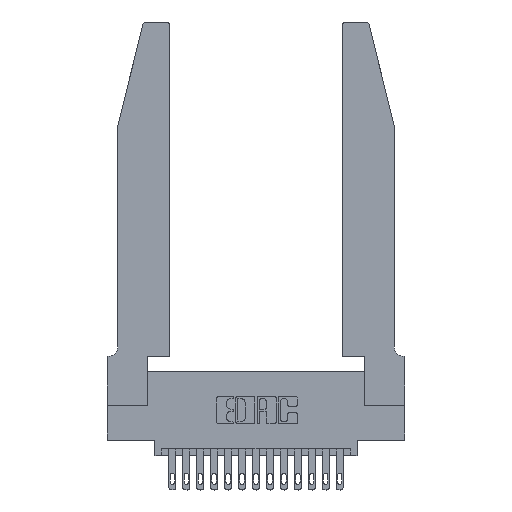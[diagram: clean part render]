
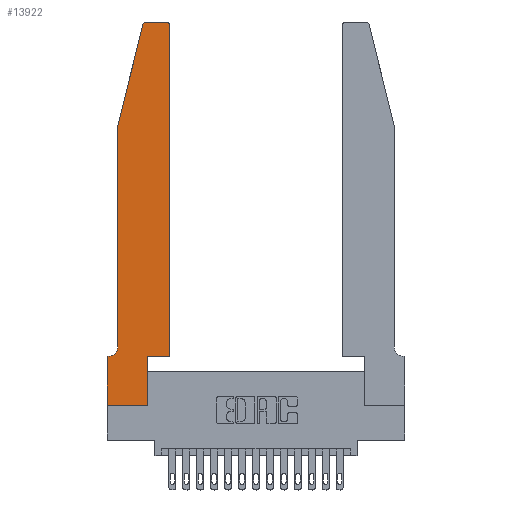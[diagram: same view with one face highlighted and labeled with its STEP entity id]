
A CAD part, top view. The second image highlights one B-rep face of the part: STEP entity #13922.
In plain terms, the highlighted planar face has unit normal (0, 0, 1).
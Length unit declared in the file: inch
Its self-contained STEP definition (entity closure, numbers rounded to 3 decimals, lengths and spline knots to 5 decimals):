
#42 = CARTESIAN_POINT ( 'NONE',  ( 0.25487, 2.72718, 0.37 ) ) ;
#198 = EDGE_LOOP ( 'NONE', ( #1298, #3548, #8835, #11519, #1738, #9997, #5464, #5388, #15684, #5136, #5292, #12281 ) ) ;
#418 = CARTESIAN_POINT ( 'NONE',  ( 0.0755, 2., 0.37 ) ) ;
#589 = VECTOR ( 'NONE', #10722, 39.37008 ) ;
#644 = VERTEX_POINT ( 'NONE', #4199 ) ;
#688 = VERTEX_POINT ( 'NONE', #10249 ) ;
#1087 = DIRECTION ( 'NONE',  ( 0., -1., 0. ) ) ;
#1140 = CARTESIAN_POINT ( 'NONE',  ( 0.4505, 0.35, 0.37 ) ) ;
#1259 = LINE ( 'NONE', #418, #589 ) ;
#1298 = ORIENTED_EDGE ( 'NONE', *, *, #5719, .T. ) ;
#1547 = AXIS2_PLACEMENT_3D ( 'NONE', #6113, #16188, #14755 ) ;
#1638 = LINE ( 'NONE', #12558, #17407 ) ;
#1664 = VECTOR ( 'NONE', #8666, 39.37008 ) ;
#1738 = ORIENTED_EDGE ( 'NONE', *, *, #2951, .T. ) ;
#1989 = CARTESIAN_POINT ( 'NONE',  ( 0.284, 2.75, 0.37 ) ) ;
#2195 = CARTESIAN_POINT ( 'NONE',  ( 0.0055, 0.42, 0.37 ) ) ;
#2221 = VERTEX_POINT ( 'NONE', #42 ) ;
#2312 = DIRECTION ( 'NONE',  ( -1., 0., 0. ) ) ;
#2484 = EDGE_CURVE ( 'NONE', #2221, #11481, #15965, .T. ) ;
#2888 = VERTEX_POINT ( 'NONE', #13269 ) ;
#2951 = EDGE_CURVE ( 'NONE', #7596, #6739, #17776, .T. ) ;
#3108 = AXIS2_PLACEMENT_3D ( 'NONE', #17528, #14323, #4329 ) ;
#3548 = ORIENTED_EDGE ( 'NONE', *, *, #6432, .T. ) ;
#3698 = CARTESIAN_POINT ( 'NONE',  ( 0.0755, 2., 0.37 ) ) ;
#3859 = CARTESIAN_POINT ( 'NONE',  ( 0., 0., 0.37 ) ) ;
#3917 = AXIS2_PLACEMENT_3D ( 'NONE', #2195, #6476, #2312 ) ;
#4199 = CARTESIAN_POINT ( 'NONE',  ( 0.2865, 0., 0.37 ) ) ;
#4329 = DIRECTION ( 'NONE',  ( 1., 0., 0. ) ) ;
#4801 = PLANE ( 'NONE',  #12770 ) ;
#4879 = LINE ( 'NONE', #15777, #10880 ) ;
#5136 = ORIENTED_EDGE ( 'NONE', *, *, #18772, .T. ) ;
#5223 = DIRECTION ( 'NONE',  ( 0., 1., 0. ) ) ;
#5292 = ORIENTED_EDGE ( 'NONE', *, *, #9496, .T. ) ;
#5388 = ORIENTED_EDGE ( 'NONE', *, *, #17598, .T. ) ;
#5464 = ORIENTED_EDGE ( 'NONE', *, *, #12644, .T. ) ;
#5689 = DIRECTION ( 'NONE',  ( 1., 0., 0. ) ) ;
#5719 = EDGE_CURVE ( 'NONE', #17930, #8966, #15848, .T. ) ;
#5750 = VERTEX_POINT ( 'NONE', #3859 ) ;
#6113 = CARTESIAN_POINT ( 'NONE',  ( 0.284, 2.72, 0.37 ) ) ;
#6161 = CARTESIAN_POINT ( 'NONE',  ( 0., 0.35, 0.37 ) ) ;
#6290 = EDGE_CURVE ( 'NONE', #14970, #17930, #12743, .T. ) ;
#6298 = CARTESIAN_POINT ( 'NONE',  ( 0.4205, 2.75, 0.37 ) ) ;
#6432 = EDGE_CURVE ( 'NONE', #8966, #2221, #9104, .T. ) ;
#6476 = DIRECTION ( 'NONE',  ( 0., 0., -1. ) ) ;
#6550 = EDGE_CURVE ( 'NONE', #644, #688, #17522, .T. ) ;
#6739 = VERTEX_POINT ( 'NONE', #7334 ) ;
#6875 = CARTESIAN_POINT ( 'NONE',  ( 0.4505, 2.72, 0.37 ) ) ;
#7334 = CARTESIAN_POINT ( 'NONE',  ( 0.0055, 0.35, 0.37 ) ) ;
#7596 = VERTEX_POINT ( 'NONE', #17418 ) ;
#7717 = FACE_OUTER_BOUND ( 'NONE', #198, .T. ) ;
#7794 = DIRECTION ( 'NONE',  ( 0., 0., 1. ) ) ;
#7965 = LINE ( 'NONE', #8458, #18677 ) ;
#8413 = CARTESIAN_POINT ( 'NONE',  ( 0.2605, 2.75, 0.37 ) ) ;
#8458 = CARTESIAN_POINT ( 'NONE',  ( 0., 0., 0.37 ) ) ;
#8666 = DIRECTION ( 'NONE',  ( 1., 0., 0. ) ) ;
#8835 = ORIENTED_EDGE ( 'NONE', *, *, #2484, .T. ) ;
#8966 = VERTEX_POINT ( 'NONE', #1989 ) ;
#9104 = CIRCLE ( 'NONE', #1547, 0.03 ) ;
#9456 = CARTESIAN_POINT ( 'NONE',  ( 0.0755, 2., 0.37 ) ) ;
#9486 = DIRECTION ( 'NONE',  ( -0.239, -0.971, 0. ) ) ;
#9496 = EDGE_CURVE ( 'NONE', #18147, #14970, #1638, .T. ) ;
#9997 = ORIENTED_EDGE ( 'NONE', *, *, #16206, .T. ) ;
#10249 = CARTESIAN_POINT ( 'NONE',  ( 0.2865, 0.35, 0.37 ) ) ;
#10722 = DIRECTION ( 'NONE',  ( 0., -1., 0. ) ) ;
#10880 = VECTOR ( 'NONE', #13082, 39.37008 ) ;
#11481 = VERTEX_POINT ( 'NONE', #9456 ) ;
#11519 = ORIENTED_EDGE ( 'NONE', *, *, #16263, .T. ) ;
#11598 = CARTESIAN_POINT ( 'NONE',  ( 0.2865, 0.35, 0.37 ) ) ;
#11915 = LINE ( 'NONE', #15937, #18776 ) ;
#12281 = ORIENTED_EDGE ( 'NONE', *, *, #6290, .T. ) ;
#12558 = CARTESIAN_POINT ( 'NONE',  ( 0.4505, 0.35, 0.37 ) ) ;
#12644 = EDGE_CURVE ( 'NONE', #2888, #5750, #7965, .T. ) ;
#12662 = VECTOR ( 'NONE', #15522, 39.37008 ) ;
#12743 = CIRCLE ( 'NONE', #3108, 0.03 ) ;
#12770 = AXIS2_PLACEMENT_3D ( 'NONE', #6161, #7794, #14939 ) ;
#13082 = DIRECTION ( 'NONE',  ( -1., 0., 0. ) ) ;
#13269 = CARTESIAN_POINT ( 'NONE',  ( 0., 0.35, 0.37 ) ) ;
#13784 = LINE ( 'NONE', #14622, #1664 ) ;
#13922 = ADVANCED_FACE ( 'NONE', ( #7717 ), #4801, .T. ) ;
#14323 = DIRECTION ( 'NONE',  ( 0., 0., 1. ) ) ;
#14622 = CARTESIAN_POINT ( 'NONE',  ( 0., 0., 0.37 ) ) ;
#14755 = DIRECTION ( 'NONE',  ( 1., 0., 0. ) ) ;
#14939 = DIRECTION ( 'NONE',  ( 1., 0., 0. ) ) ;
#14970 = VERTEX_POINT ( 'NONE', #6875 ) ;
#15458 = VECTOR ( 'NONE', #17602, 39.37008 ) ;
#15522 = DIRECTION ( 'NONE',  ( -1., 0., 0. ) ) ;
#15684 = ORIENTED_EDGE ( 'NONE', *, *, #6550, .T. ) ;
#15777 = CARTESIAN_POINT ( 'NONE',  ( 0.0755, 0.35, 0.37 ) ) ;
#15848 = LINE ( 'NONE', #8413, #12662 ) ;
#15937 = CARTESIAN_POINT ( 'NONE',  ( 0.4505, 0.35, 0.37 ) ) ;
#15965 = LINE ( 'NONE', #3698, #17556 ) ;
#16188 = DIRECTION ( 'NONE',  ( 0., 0., 1. ) ) ;
#16206 = EDGE_CURVE ( 'NONE', #6739, #2888, #4879, .T. ) ;
#16263 = EDGE_CURVE ( 'NONE', #11481, #7596, #1259, .T. ) ;
#17407 = VECTOR ( 'NONE', #5223, 39.37008 ) ;
#17418 = CARTESIAN_POINT ( 'NONE',  ( 0.0755, 0.42, 0.37 ) ) ;
#17522 = LINE ( 'NONE', #11598, #15458 ) ;
#17528 = CARTESIAN_POINT ( 'NONE',  ( 0.4205, 2.72, 0.37 ) ) ;
#17556 = VECTOR ( 'NONE', #9486, 39.37008 ) ;
#17598 = EDGE_CURVE ( 'NONE', #5750, #644, #13784, .T. ) ;
#17602 = DIRECTION ( 'NONE',  ( 0., 1., 0. ) ) ;
#17776 = CIRCLE ( 'NONE', #3917, 0.07 ) ;
#17930 = VERTEX_POINT ( 'NONE', #6298 ) ;
#18147 = VERTEX_POINT ( 'NONE', #1140 ) ;
#18677 = VECTOR ( 'NONE', #1087, 39.37008 ) ;
#18772 = EDGE_CURVE ( 'NONE', #688, #18147, #11915, .T. ) ;
#18776 = VECTOR ( 'NONE', #5689, 39.37008 ) ;
